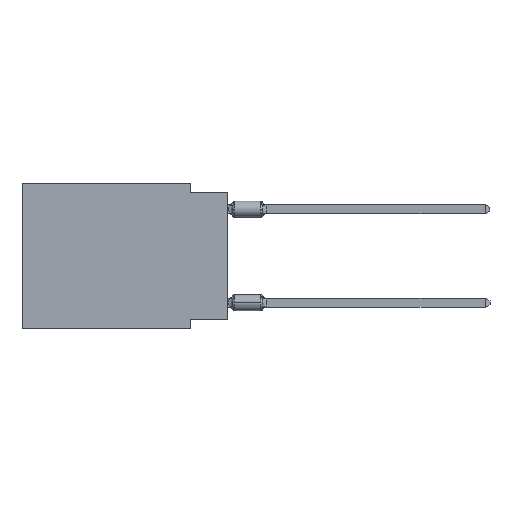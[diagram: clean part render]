
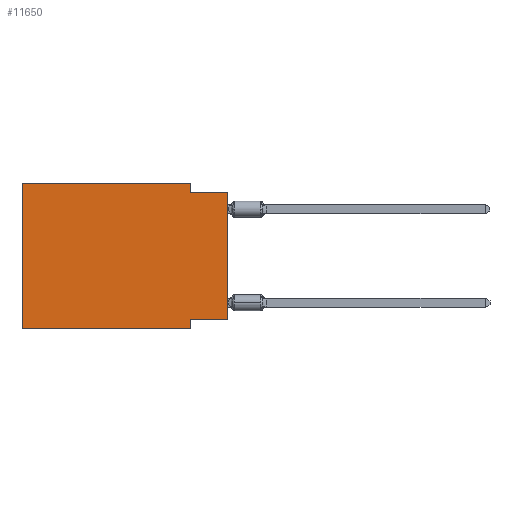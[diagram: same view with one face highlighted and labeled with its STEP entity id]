
A CAD part, left-side view. The second image highlights one B-rep face of the part: STEP entity #11650.
In plain terms, the highlighted planar face has unit normal (-1, 0, 0).
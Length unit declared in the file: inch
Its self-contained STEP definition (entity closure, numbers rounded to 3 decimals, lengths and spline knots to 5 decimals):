
#27 = ORIENTED_EDGE ( 'NONE', *, *, #7310, .T. ) ;
#117 = CARTESIAN_POINT ( 'NONE',  ( 0., 0., 0. ) ) ;
#144 = VECTOR ( 'NONE', #12708, 39.37008 ) ;
#344 = EDGE_CURVE ( 'NONE', #3089, #9645, #7968, .T. ) ;
#438 = VECTOR ( 'NONE', #1867, 39.37008 ) ;
#1189 = ORIENTED_EDGE ( 'NONE', *, *, #11074, .F. ) ;
#1211 = CARTESIAN_POINT ( 'NONE',  ( 0., 0.1, -0.39 ) ) ;
#1336 = FACE_OUTER_BOUND ( 'NONE', #9651, .T. ) ;
#1533 = CARTESIAN_POINT ( 'NONE',  ( 0., 0.55, 0. ) ) ;
#1575 = CARTESIAN_POINT ( 'NONE',  ( 0., 0.1, 0. ) ) ;
#1683 = DIRECTION ( 'NONE',  ( 0., -1., 0. ) ) ;
#1867 = DIRECTION ( 'NONE',  ( 0., -1., 0. ) ) ;
#2456 = VECTOR ( 'NONE', #5460, 39.37008 ) ;
#2896 = CARTESIAN_POINT ( 'NONE',  ( 0., 0., -0.365 ) ) ;
#3089 = VERTEX_POINT ( 'NONE', #11707 ) ;
#3308 = VECTOR ( 'NONE', #11134, 39.37008 ) ;
#3484 = VECTOR ( 'NONE', #4581, 39.37008 ) ;
#3500 = CARTESIAN_POINT ( 'NONE',  ( 0., 0., -0.025 ) ) ;
#3515 = DIRECTION ( 'NONE',  ( 0., 0., -1. ) ) ;
#3535 = CARTESIAN_POINT ( 'NONE',  ( 0., 0.1, -0.365 ) ) ;
#3651 = CARTESIAN_POINT ( 'NONE',  ( 0., 0.55, 0. ) ) ;
#3781 = EDGE_CURVE ( 'NONE', #3089, #12877, #7730, .T. ) ;
#3788 = EDGE_CURVE ( 'NONE', #12877, #6279, #12513, .T. ) ;
#3807 = VECTOR ( 'NONE', #9558, 39.37008 ) ;
#3951 = ORIENTED_EDGE ( 'NONE', *, *, #8439, .F. ) ;
#4110 = EDGE_CURVE ( 'NONE', #6718, #12549, #8917, .T. ) ;
#4119 = AXIS2_PLACEMENT_3D ( 'NONE', #10528, #5283, #3515 ) ;
#4560 = ORIENTED_EDGE ( 'NONE', *, *, #3788, .F. ) ;
#4581 = DIRECTION ( 'NONE',  ( 0., -1., 0. ) ) ;
#4705 = LINE ( 'NONE', #6809, #3484 ) ;
#5019 = CARTESIAN_POINT ( 'NONE',  ( 0., 0., -0.365 ) ) ;
#5283 = DIRECTION ( 'NONE',  ( 1., 0., 0. ) ) ;
#5394 = LINE ( 'NONE', #1575, #2456 ) ;
#5460 = DIRECTION ( 'NONE',  ( 0., 0., -1. ) ) ;
#5492 = CARTESIAN_POINT ( 'NONE',  ( 0., 0.55, 0. ) ) ;
#5821 = CARTESIAN_POINT ( 'NONE',  ( 0., 0.1, -0.39 ) ) ;
#6279 = VERTEX_POINT ( 'NONE', #12972 ) ;
#6481 = PLANE ( 'NONE',  #4119 ) ;
#6718 = VERTEX_POINT ( 'NONE', #5019 ) ;
#6809 = CARTESIAN_POINT ( 'NONE',  ( 0., 0., -0.025 ) ) ;
#6867 = CARTESIAN_POINT ( 'NONE',  ( 0., 0.55, -0.39 ) ) ;
#7310 = EDGE_CURVE ( 'NONE', #6718, #11228, #10086, .T. ) ;
#7487 = ORIENTED_EDGE ( 'NONE', *, *, #9006, .F. ) ;
#7730 = LINE ( 'NONE', #5492, #3807 ) ;
#7765 = DIRECTION ( 'NONE',  ( 0., 1., 0. ) ) ;
#7968 = LINE ( 'NONE', #6867, #438 ) ;
#8132 = ORIENTED_EDGE ( 'NONE', *, *, #344, .T. ) ;
#8439 = EDGE_CURVE ( 'NONE', #12549, #9645, #8697, .T. ) ;
#8542 = VERTEX_POINT ( 'NONE', #11177 ) ;
#8697 = LINE ( 'NONE', #5821, #144 ) ;
#8917 = LINE ( 'NONE', #2896, #11350 ) ;
#9006 = EDGE_CURVE ( 'NONE', #6279, #8542, #5394, .T. ) ;
#9500 = ORIENTED_EDGE ( 'NONE', *, *, #3781, .F. ) ;
#9558 = DIRECTION ( 'NONE',  ( 0., 0., 1. ) ) ;
#9645 = VERTEX_POINT ( 'NONE', #1211 ) ;
#9651 = EDGE_LOOP ( 'NONE', ( #27, #1189, #7487, #4560, #9500, #8132, #3951, #9661 ) ) ;
#9661 = ORIENTED_EDGE ( 'NONE', *, *, #4110, .F. ) ;
#10086 = LINE ( 'NONE', #117, #3308 ) ;
#10528 = CARTESIAN_POINT ( 'NONE',  ( 0., 0.55, 0. ) ) ;
#11074 = EDGE_CURVE ( 'NONE', #8542, #11228, #4705, .T. ) ;
#11134 = DIRECTION ( 'NONE',  ( 0., 0., 1. ) ) ;
#11177 = CARTESIAN_POINT ( 'NONE',  ( 0., 0.1, -0.025 ) ) ;
#11228 = VERTEX_POINT ( 'NONE', #3500 ) ;
#11350 = VECTOR ( 'NONE', #7765, 39.37008 ) ;
#11650 = ADVANCED_FACE ( 'NONE', ( #1336 ), #6481, .F. ) ;
#11707 = CARTESIAN_POINT ( 'NONE',  ( 0., 0.55, -0.39 ) ) ;
#11772 = VECTOR ( 'NONE', #1683, 39.37008 ) ;
#12513 = LINE ( 'NONE', #3651, #11772 ) ;
#12549 = VERTEX_POINT ( 'NONE', #3535 ) ;
#12708 = DIRECTION ( 'NONE',  ( 0., 0., -1. ) ) ;
#12877 = VERTEX_POINT ( 'NONE', #1533 ) ;
#12972 = CARTESIAN_POINT ( 'NONE',  ( 0., 0.1, 0. ) ) ;
